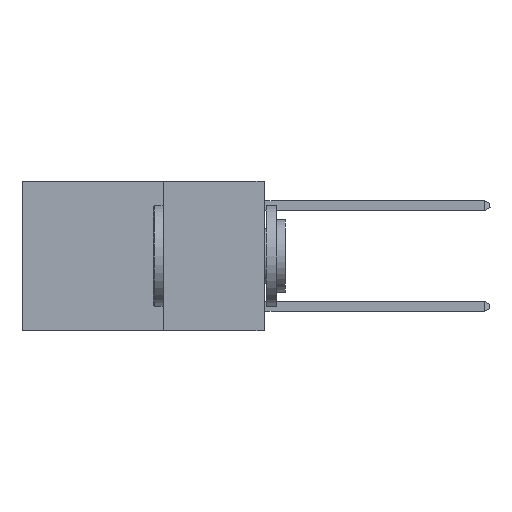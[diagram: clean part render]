
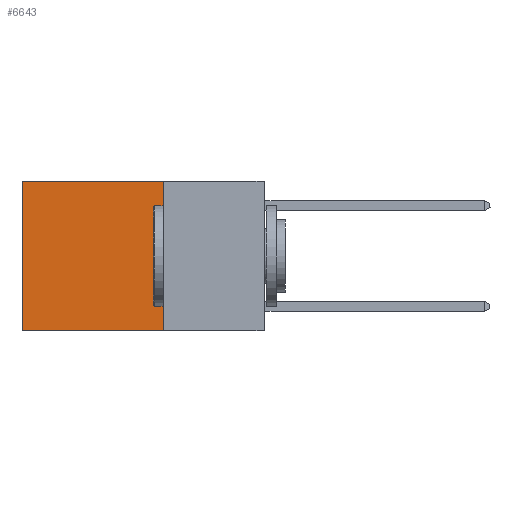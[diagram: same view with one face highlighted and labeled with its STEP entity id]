
A CAD part, left-side view. The second image highlights one B-rep face of the part: STEP entity #6643.
In plain terms, the highlighted planar face has unit normal (-1, 0, 0).
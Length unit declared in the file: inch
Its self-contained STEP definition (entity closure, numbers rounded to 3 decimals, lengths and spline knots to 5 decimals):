
#16 = VERTEX_POINT ( 'NONE', #8608 ) ;
#621 = EDGE_CURVE ( 'NONE', #16, #9446, #15759, .T. ) ;
#913 = DIRECTION ( 'NONE',  ( 0., 1., 0. ) ) ;
#1420 = CARTESIAN_POINT ( 'NONE',  ( 0.2625, 0.25, 0. ) ) ;
#1736 = ORIENTED_EDGE ( 'NONE', *, *, #621, .F. ) ;
#1831 = CARTESIAN_POINT ( 'NONE',  ( 0.2625, 0.6, 0. ) ) ;
#3156 = DIRECTION ( 'NONE',  ( 0., 0., -1. ) ) ;
#4155 = CARTESIAN_POINT ( 'NONE',  ( 0.2625, 0.25, 0. ) ) ;
#5434 = ORIENTED_EDGE ( 'NONE', *, *, #10019, .T. ) ;
#5554 = VECTOR ( 'NONE', #9433, 39.37008 ) ;
#5670 = ORIENTED_EDGE ( 'NONE', *, *, #7006, .T. ) ;
#6643 = ADVANCED_FACE ( 'NONE', ( #14349 ), #14781, .F. ) ;
#6814 = DIRECTION ( 'NONE',  ( 1., 0., 0. ) ) ;
#7006 = EDGE_CURVE ( 'NONE', #7880, #8289, #15629, .T. ) ;
#7270 = EDGE_CURVE ( 'NONE', #7880, #16, #11820, .T. ) ;
#7479 = AXIS2_PLACEMENT_3D ( 'NONE', #4155, #6814, #16150 ) ;
#7529 = CARTESIAN_POINT ( 'NONE',  ( 0.2625, 0.25, 0. ) ) ;
#7880 = VERTEX_POINT ( 'NONE', #9235 ) ;
#8289 = VERTEX_POINT ( 'NONE', #10259 ) ;
#8608 = CARTESIAN_POINT ( 'NONE',  ( 0.2625, 0.25, -0.37 ) ) ;
#8616 = VECTOR ( 'NONE', #3156, 39.37008 ) ;
#8798 = CARTESIAN_POINT ( 'NONE',  ( 0.2625, 0.25, -0.37 ) ) ;
#9235 = CARTESIAN_POINT ( 'NONE',  ( 0.2625, 0.25, 0. ) ) ;
#9323 = ORIENTED_EDGE ( 'NONE', *, *, #7270, .F. ) ;
#9433 = DIRECTION ( 'NONE',  ( 0., 1., 0. ) ) ;
#9446 = VERTEX_POINT ( 'NONE', #11386 ) ;
#10019 = EDGE_CURVE ( 'NONE', #8289, #9446, #12113, .T. ) ;
#10259 = CARTESIAN_POINT ( 'NONE',  ( 0.2625, 0.6, 0. ) ) ;
#11386 = CARTESIAN_POINT ( 'NONE',  ( 0.2625, 0.6, -0.37 ) ) ;
#11820 = LINE ( 'NONE', #1420, #14976 ) ;
#11994 = DIRECTION ( 'NONE',  ( 0., 0., -1. ) ) ;
#12113 = LINE ( 'NONE', #1831, #8616 ) ;
#12471 = VECTOR ( 'NONE', #913, 39.37008 ) ;
#14349 = FACE_OUTER_BOUND ( 'NONE', #16214, .T. ) ;
#14781 = PLANE ( 'NONE',  #7479 ) ;
#14976 = VECTOR ( 'NONE', #11994, 39.37008 ) ;
#15629 = LINE ( 'NONE', #7529, #12471 ) ;
#15759 = LINE ( 'NONE', #8798, #5554 ) ;
#16150 = DIRECTION ( 'NONE',  ( 0., 0., -1. ) ) ;
#16214 = EDGE_LOOP ( 'NONE', ( #5434, #1736, #9323, #5670 ) ) ;
